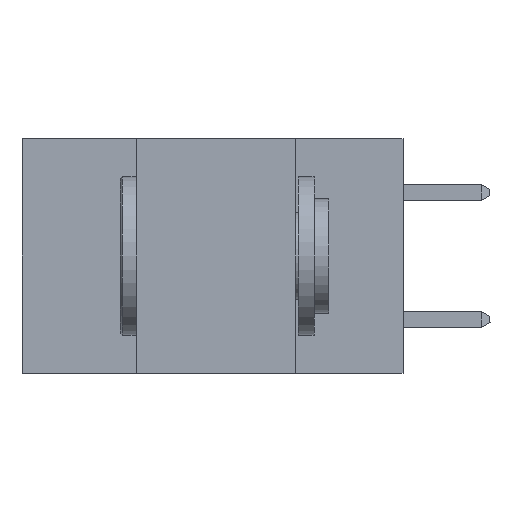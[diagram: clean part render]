
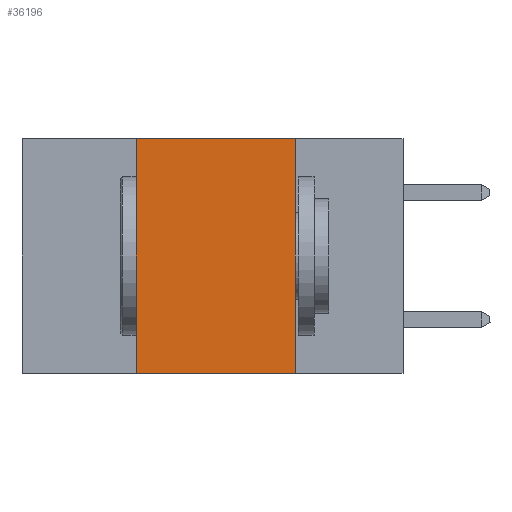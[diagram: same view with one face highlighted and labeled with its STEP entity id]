
A CAD part, left-side view. The second image highlights one B-rep face of the part: STEP entity #36196.
In plain terms, the highlighted planar face has unit normal (-1, 0, 0).
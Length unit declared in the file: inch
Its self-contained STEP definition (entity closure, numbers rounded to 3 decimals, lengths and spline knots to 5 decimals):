
#1234 = CARTESIAN_POINT ( 'NONE',  ( 0., 0.6, 0. ) ) ;
#2648 = EDGE_LOOP ( 'NONE', ( #37128, #36672, #8791, #36698 ) ) ;
#2984 = LINE ( 'NONE', #4533, #37577 ) ;
#4533 = CARTESIAN_POINT ( 'NONE',  ( 0., 0.42, 0. ) ) ;
#4591 = PLANE ( 'NONE',  #22180 ) ;
#6456 = CARTESIAN_POINT ( 'NONE',  ( 0., 0.6, 0. ) ) ;
#7873 = DIRECTION ( 'NONE',  ( 0., 0., -1. ) ) ;
#8791 = ORIENTED_EDGE ( 'NONE', *, *, #12924, .F. ) ;
#9688 = VECTOR ( 'NONE', #38967, 39.37008 ) ;
#9701 = CARTESIAN_POINT ( 'NONE',  ( 0., 0.6, -0.37 ) ) ;
#11054 = DIRECTION ( 'NONE',  ( 1., 0., 0. ) ) ;
#12251 = CARTESIAN_POINT ( 'NONE',  ( 0., 0.42, -0.37 ) ) ;
#12924 = EDGE_CURVE ( 'NONE', #29889, #24966, #2984, .T. ) ;
#14038 = VECTOR ( 'NONE', #33909, 39.37008 ) ;
#14526 = CARTESIAN_POINT ( 'NONE',  ( 0., 0.17, 0. ) ) ;
#15304 = EDGE_CURVE ( 'NONE', #34974, #16467, #21608, .T. ) ;
#16467 = VERTEX_POINT ( 'NONE', #23051 ) ;
#17274 = LINE ( 'NONE', #6456, #9688 ) ;
#21218 = EDGE_CURVE ( 'NONE', #24966, #34974, #17274, .T. ) ;
#21608 = LINE ( 'NONE', #14526, #14038 ) ;
#21861 = EDGE_CURVE ( 'NONE', #29889, #16467, #33924, .T. ) ;
#22180 = AXIS2_PLACEMENT_3D ( 'NONE', #1234, #11054, #7873 ) ;
#23051 = CARTESIAN_POINT ( 'NONE',  ( 0., 0.17, -0.37 ) ) ;
#23964 = DIRECTION ( 'NONE',  ( 0., 0., 1. ) ) ;
#24966 = VERTEX_POINT ( 'NONE', #31724 ) ;
#25300 = VECTOR ( 'NONE', #25805, 39.37008 ) ;
#25345 = CARTESIAN_POINT ( 'NONE',  ( 0., 0.17, 0. ) ) ;
#25805 = DIRECTION ( 'NONE',  ( 0., -1., 0. ) ) ;
#28068 = FACE_OUTER_BOUND ( 'NONE', #2648, .T. ) ;
#29889 = VERTEX_POINT ( 'NONE', #12251 ) ;
#31724 = CARTESIAN_POINT ( 'NONE',  ( 0., 0.42, 0. ) ) ;
#33909 = DIRECTION ( 'NONE',  ( 0., 0., -1. ) ) ;
#33924 = LINE ( 'NONE', #9701, #25300 ) ;
#34974 = VERTEX_POINT ( 'NONE', #25345 ) ;
#36196 = ADVANCED_FACE ( 'NONE', ( #28068 ), #4591, .F. ) ;
#36672 = ORIENTED_EDGE ( 'NONE', *, *, #21218, .F. ) ;
#36698 = ORIENTED_EDGE ( 'NONE', *, *, #21861, .T. ) ;
#37128 = ORIENTED_EDGE ( 'NONE', *, *, #15304, .F. ) ;
#37577 = VECTOR ( 'NONE', #23964, 39.37008 ) ;
#38967 = DIRECTION ( 'NONE',  ( 0., -1., 0. ) ) ;
